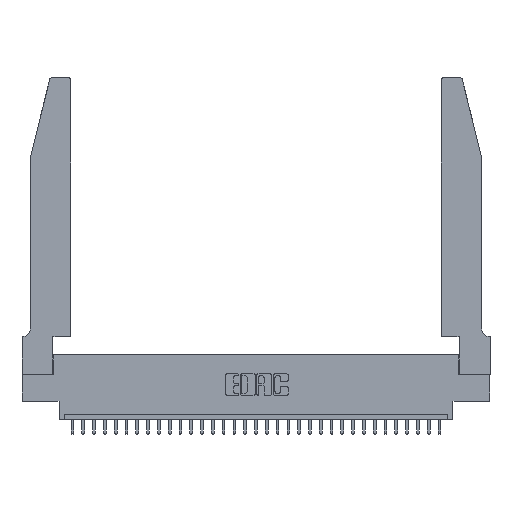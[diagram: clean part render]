
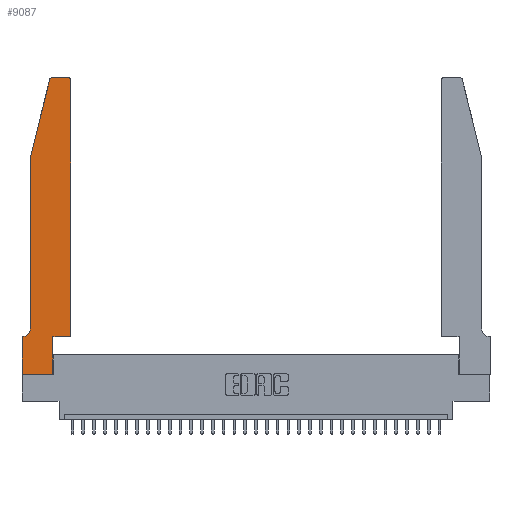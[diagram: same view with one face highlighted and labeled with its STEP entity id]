
A CAD part, top view. The second image highlights one B-rep face of the part: STEP entity #9087.
In plain terms, the highlighted planar face has unit normal (0, 0, 1).
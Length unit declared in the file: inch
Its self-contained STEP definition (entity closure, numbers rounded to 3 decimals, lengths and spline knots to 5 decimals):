
#99 = CARTESIAN_POINT ( 'NONE',  ( 0.4205, 2.72, 0.37 ) ) ;
#415 = CARTESIAN_POINT ( 'NONE',  ( 0.284, 2.75, 0.37 ) ) ;
#1349 = CARTESIAN_POINT ( 'NONE',  ( 0.4505, 0.35, 0.37 ) ) ;
#1350 = CARTESIAN_POINT ( 'NONE',  ( 0.284, 2.72, 0.37 ) ) ;
#1912 = CARTESIAN_POINT ( 'NONE',  ( 0., 0., 0.37 ) ) ;
#2227 = DIRECTION ( 'NONE',  ( 0., 0., 1. ) ) ;
#2877 = VECTOR ( 'NONE', #5499, 39.37008 ) ;
#3047 = ORIENTED_EDGE ( 'NONE', *, *, #15589, .T. ) ;
#3170 = CARTESIAN_POINT ( 'NONE',  ( 0., 0.35, 0.37 ) ) ;
#3800 = VECTOR ( 'NONE', #22280, 39.37008 ) ;
#4106 = CARTESIAN_POINT ( 'NONE',  ( 0.2865, 0.35, 0.37 ) ) ;
#4852 = ORIENTED_EDGE ( 'NONE', *, *, #32036, .T. ) ;
#4909 = VECTOR ( 'NONE', #17593, 39.37008 ) ;
#5115 = AXIS2_PLACEMENT_3D ( 'NONE', #16969, #2227, #12699 ) ;
#5212 = VECTOR ( 'NONE', #23358, 39.37008 ) ;
#5265 = DIRECTION ( 'NONE',  ( 1., 0., 0. ) ) ;
#5499 = DIRECTION ( 'NONE',  ( -1., 0., 0. ) ) ;
#6392 = DIRECTION ( 'NONE',  ( 0., -1., 0. ) ) ;
#6627 = VERTEX_POINT ( 'NONE', #1912 ) ;
#6713 = CARTESIAN_POINT ( 'NONE',  ( 0., 0., 0.37 ) ) ;
#6828 = EDGE_CURVE ( 'NONE', #19456, #16219, #27974, .T. ) ;
#7257 = ORIENTED_EDGE ( 'NONE', *, *, #19609, .T. ) ;
#7584 = FACE_OUTER_BOUND ( 'NONE', #25390, .T. ) ;
#7609 = DIRECTION ( 'NONE',  ( 0., 1., 0. ) ) ;
#7704 = LINE ( 'NONE', #21284, #12724 ) ;
#7806 = CIRCLE ( 'NONE', #17708, 0.07 ) ;
#8070 = AXIS2_PLACEMENT_3D ( 'NONE', #99, #17670, #5265 ) ;
#8239 = EDGE_CURVE ( 'NONE', #31811, #18444, #25533, .T. ) ;
#8240 = CARTESIAN_POINT ( 'NONE',  ( 0.4505, 0.35, 0.37 ) ) ;
#8828 = LINE ( 'NONE', #15053, #4909 ) ;
#9087 = ADVANCED_FACE ( 'NONE', ( #7584 ), #31999, .T. ) ;
#9254 = ORIENTED_EDGE ( 'NONE', *, *, #21902, .T. ) ;
#9261 = CARTESIAN_POINT ( 'NONE',  ( 0.2605, 2.75, 0.37 ) ) ;
#10570 = ORIENTED_EDGE ( 'NONE', *, *, #6828, .T. ) ;
#10883 = VERTEX_POINT ( 'NONE', #19213 ) ;
#11012 = CARTESIAN_POINT ( 'NONE',  ( 0.4505, 0.35, 0.37 ) ) ;
#11264 = CARTESIAN_POINT ( 'NONE',  ( 0.25487, 2.72718, 0.37 ) ) ;
#11582 = VECTOR ( 'NONE', #14168, 39.37008 ) ;
#12559 = VERTEX_POINT ( 'NONE', #31784 ) ;
#12687 = LINE ( 'NONE', #19762, #3800 ) ;
#12699 = DIRECTION ( 'NONE',  ( 1., 0., 0. ) ) ;
#12724 = VECTOR ( 'NONE', #6392, 39.37008 ) ;
#13571 = CARTESIAN_POINT ( 'NONE',  ( 0.0055, 0.42, 0.37 ) ) ;
#14168 = DIRECTION ( 'NONE',  ( 0., -1., 0. ) ) ;
#15053 = CARTESIAN_POINT ( 'NONE',  ( 0., 0., 0.37 ) ) ;
#15291 = EDGE_CURVE ( 'NONE', #19454, #31811, #26069, .T. ) ;
#15529 = ORIENTED_EDGE ( 'NONE', *, *, #25483, .T. ) ;
#15589 = EDGE_CURVE ( 'NONE', #17486, #12559, #7704, .T. ) ;
#16051 = LINE ( 'NONE', #25418, #2877 ) ;
#16219 = VERTEX_POINT ( 'NONE', #11012 ) ;
#16298 = DIRECTION ( 'NONE',  ( 1., 0., 0. ) ) ;
#16969 = CARTESIAN_POINT ( 'NONE',  ( 0., 0.35, 0.37 ) ) ;
#17486 = VERTEX_POINT ( 'NONE', #18267 ) ;
#17593 = DIRECTION ( 'NONE',  ( 1., 0., 0. ) ) ;
#17670 = DIRECTION ( 'NONE',  ( 0., 0., 1. ) ) ;
#17708 = AXIS2_PLACEMENT_3D ( 'NONE', #13571, #18383, #23411 ) ;
#17718 = EDGE_CURVE ( 'NONE', #10883, #27302, #16051, .T. ) ;
#18267 = CARTESIAN_POINT ( 'NONE',  ( 0.0755, 2., 0.37 ) ) ;
#18383 = DIRECTION ( 'NONE',  ( 0., 0., -1. ) ) ;
#18444 = VERTEX_POINT ( 'NONE', #415 ) ;
#19213 = CARTESIAN_POINT ( 'NONE',  ( 0.0055, 0.35, 0.37 ) ) ;
#19454 = VERTEX_POINT ( 'NONE', #31267 ) ;
#19456 = VERTEX_POINT ( 'NONE', #4106 ) ;
#19609 = EDGE_CURVE ( 'NONE', #12559, #10883, #7806, .T. ) ;
#19762 = CARTESIAN_POINT ( 'NONE',  ( 0.0755, 2., 0.37 ) ) ;
#19815 = ORIENTED_EDGE ( 'NONE', *, *, #30379, .T. ) ;
#20024 = VECTOR ( 'NONE', #7609, 39.37008 ) ;
#20832 = LINE ( 'NONE', #29190, #20024 ) ;
#21104 = CARTESIAN_POINT ( 'NONE',  ( 0.2865, 0., 0.37 ) ) ;
#21284 = CARTESIAN_POINT ( 'NONE',  ( 0.0755, 2., 0.37 ) ) ;
#21364 = VECTOR ( 'NONE', #31753, 39.37008 ) ;
#21902 = EDGE_CURVE ( 'NONE', #6627, #25371, #8828, .T. ) ;
#22218 = ORIENTED_EDGE ( 'NONE', *, *, #17718, .T. ) ;
#22280 = DIRECTION ( 'NONE',  ( -0.239, -0.971, 0. ) ) ;
#22385 = CARTESIAN_POINT ( 'NONE',  ( 0.4205, 2.75, 0.37 ) ) ;
#23082 = ORIENTED_EDGE ( 'NONE', *, *, #29438, .T. ) ;
#23213 = ORIENTED_EDGE ( 'NONE', *, *, #8239, .T. ) ;
#23358 = DIRECTION ( 'NONE',  ( 0., 1., 0. ) ) ;
#23411 = DIRECTION ( 'NONE',  ( -1., 0., 0. ) ) ;
#23865 = DIRECTION ( 'NONE',  ( -1., 0., 0. ) ) ;
#24003 = VERTEX_POINT ( 'NONE', #11264 ) ;
#24726 = LINE ( 'NONE', #8240, #5212 ) ;
#24773 = VECTOR ( 'NONE', #23865, 39.37008 ) ;
#25108 = ORIENTED_EDGE ( 'NONE', *, *, #26281, .T. ) ;
#25290 = CIRCLE ( 'NONE', #27499, 0.03 ) ;
#25371 = VERTEX_POINT ( 'NONE', #21104 ) ;
#25390 = EDGE_LOOP ( 'NONE', ( #23213, #23082, #15529, #3047, #7257, #22218, #19815, #9254, #25108, #10570, #4852, #30850 ) ) ;
#25418 = CARTESIAN_POINT ( 'NONE',  ( 0.0755, 0.35, 0.37 ) ) ;
#25483 = EDGE_CURVE ( 'NONE', #24003, #17486, #12687, .T. ) ;
#25533 = LINE ( 'NONE', #9261, #24773 ) ;
#25590 = LINE ( 'NONE', #6713, #11582 ) ;
#25899 = DIRECTION ( 'NONE',  ( 0., 0., 1. ) ) ;
#26069 = CIRCLE ( 'NONE', #8070, 0.03 ) ;
#26281 = EDGE_CURVE ( 'NONE', #25371, #19456, #20832, .T. ) ;
#27302 = VERTEX_POINT ( 'NONE', #3170 ) ;
#27499 = AXIS2_PLACEMENT_3D ( 'NONE', #1350, #25899, #16298 ) ;
#27974 = LINE ( 'NONE', #1349, #21364 ) ;
#29190 = CARTESIAN_POINT ( 'NONE',  ( 0.2865, 0.35, 0.37 ) ) ;
#29438 = EDGE_CURVE ( 'NONE', #18444, #24003, #25290, .T. ) ;
#30379 = EDGE_CURVE ( 'NONE', #27302, #6627, #25590, .T. ) ;
#30850 = ORIENTED_EDGE ( 'NONE', *, *, #15291, .T. ) ;
#31267 = CARTESIAN_POINT ( 'NONE',  ( 0.4505, 2.72, 0.37 ) ) ;
#31753 = DIRECTION ( 'NONE',  ( 1., 0., 0. ) ) ;
#31784 = CARTESIAN_POINT ( 'NONE',  ( 0.0755, 0.42, 0.37 ) ) ;
#31811 = VERTEX_POINT ( 'NONE', #22385 ) ;
#31999 = PLANE ( 'NONE',  #5115 ) ;
#32036 = EDGE_CURVE ( 'NONE', #16219, #19454, #24726, .T. ) ;
